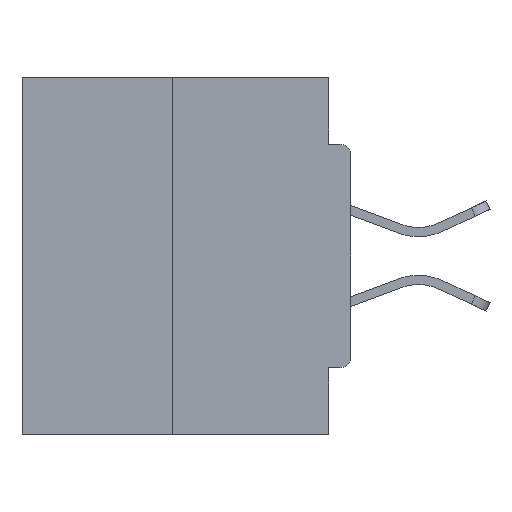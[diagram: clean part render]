
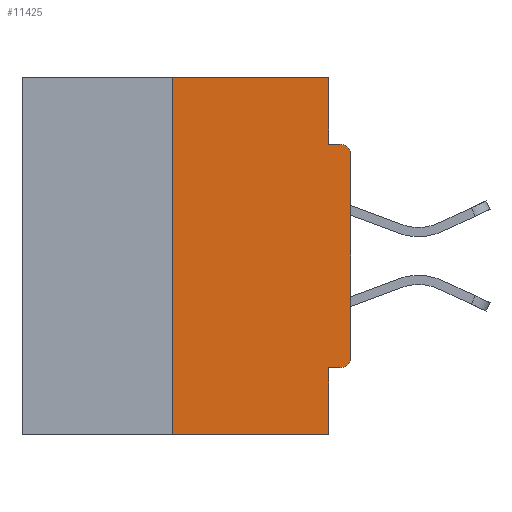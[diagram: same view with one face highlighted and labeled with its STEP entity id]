
A CAD part, left-side view. The second image highlights one B-rep face of the part: STEP entity #11425.
In plain terms, the highlighted planar face has unit normal (-1, 0, 0).
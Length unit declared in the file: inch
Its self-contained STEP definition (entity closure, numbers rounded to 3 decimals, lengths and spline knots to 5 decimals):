
#90 = VECTOR ( 'NONE', #6408, 39.37008 ) ;
#317 = ORIENTED_EDGE ( 'NONE', *, *, #34206, .F. ) ;
#780 = CARTESIAN_POINT ( 'NONE',  ( 0., 0.46, -0.5 ) ) ;
#1138 = VERTEX_POINT ( 'NONE', #7384 ) ;
#1147 = ORIENTED_EDGE ( 'NONE', *, *, #26222, .F. ) ;
#1891 = DIRECTION ( 'NONE',  ( 0., 0., 1. ) ) ;
#2937 = ORIENTED_EDGE ( 'NONE', *, *, #33532, .F. ) ;
#2979 = CARTESIAN_POINT ( 'NONE',  ( 0., 0.031, 0. ) ) ;
#3731 = LINE ( 'NONE', #7163, #4627 ) ;
#4180 = CARTESIAN_POINT ( 'NONE',  ( 0., 0.25, 0. ) ) ;
#4627 = VECTOR ( 'NONE', #1891, 39.37008 ) ;
#4870 = CARTESIAN_POINT ( 'NONE',  ( 0., 0.031, -0.4065 ) ) ;
#6396 = CARTESIAN_POINT ( 'NONE',  ( 0., 0.25, 0. ) ) ;
#6408 = DIRECTION ( 'NONE',  ( 0., -1., 0. ) ) ;
#6443 = DIRECTION ( 'NONE',  ( -1., 0., 0. ) ) ;
#6802 = DIRECTION ( 'NONE',  ( -1., 0., 0. ) ) ;
#7076 = VECTOR ( 'NONE', #23935, 39.37008 ) ;
#7163 = CARTESIAN_POINT ( 'NONE',  ( 0., 0., 0. ) ) ;
#7384 = CARTESIAN_POINT ( 'NONE',  ( 0., 0.25, -0.5 ) ) ;
#7463 = VECTOR ( 'NONE', #34844, 39.37008 ) ;
#7522 = LINE ( 'NONE', #31357, #90 ) ;
#7683 = ORIENTED_EDGE ( 'NONE', *, *, #14122, .T. ) ;
#8626 = EDGE_LOOP ( 'NONE', ( #9419, #317, #7683, #2937, #1147, #29762, #15945, #11208, #21785, #34174 ) ) ;
#8870 = EDGE_CURVE ( 'NONE', #30304, #31347, #3731, .T. ) ;
#8984 = CARTESIAN_POINT ( 'NONE',  ( 0., 0.031, -0.5 ) ) ;
#9339 = DIRECTION ( 'NONE',  ( 0., -1., 0. ) ) ;
#9419 = ORIENTED_EDGE ( 'NONE', *, *, #9723, .F. ) ;
#9717 = PLANE ( 'NONE',  #11985 ) ;
#9723 = EDGE_CURVE ( 'NONE', #26478, #11800, #12418, .T. ) ;
#10567 = CARTESIAN_POINT ( 'NONE',  ( 0., 0., -0.1085 ) ) ;
#10969 = CARTESIAN_POINT ( 'NONE',  ( 0., 0.015, -0.4065 ) ) ;
#10970 = LINE ( 'NONE', #30749, #25706 ) ;
#11057 = VERTEX_POINT ( 'NONE', #23684 ) ;
#11165 = VERTEX_POINT ( 'NONE', #10969 ) ;
#11208 = ORIENTED_EDGE ( 'NONE', *, *, #15128, .T. ) ;
#11425 = ADVANCED_FACE ( 'NONE', ( #17236 ), #9717, .F. ) ;
#11610 = CARTESIAN_POINT ( 'NONE',  ( 0., 0.031, 0. ) ) ;
#11800 = VERTEX_POINT ( 'NONE', #2979 ) ;
#11930 = CARTESIAN_POINT ( 'NONE',  ( 0., 0.015, -0.1085 ) ) ;
#11985 = AXIS2_PLACEMENT_3D ( 'NONE', #29256, #34636, #34876 ) ;
#12418 = LINE ( 'NONE', #28863, #19386 ) ;
#13959 = VECTOR ( 'NONE', #22725, 39.37008 ) ;
#14076 = EDGE_CURVE ( 'NONE', #33112, #11057, #7522, .T. ) ;
#14096 = VERTEX_POINT ( 'NONE', #8984 ) ;
#14122 = EDGE_CURVE ( 'NONE', #1138, #14096, #26658, .T. ) ;
#15128 = EDGE_CURVE ( 'NONE', #31347, #11057, #35312, .T. ) ;
#15945 = ORIENTED_EDGE ( 'NONE', *, *, #8870, .T. ) ;
#17236 = FACE_OUTER_BOUND ( 'NONE', #8626, .T. ) ;
#17503 = DIRECTION ( 'NONE',  ( 0., 0., -1. ) ) ;
#19281 = VECTOR ( 'NONE', #9339, 39.37008 ) ;
#19386 = VECTOR ( 'NONE', #31204, 39.37008 ) ;
#20306 = AXIS2_PLACEMENT_3D ( 'NONE', #11930, #6443, #31748 ) ;
#21430 = LINE ( 'NONE', #29426, #7076 ) ;
#21785 = ORIENTED_EDGE ( 'NONE', *, *, #14076, .F. ) ;
#21982 = VERTEX_POINT ( 'NONE', #4870 ) ;
#22725 = DIRECTION ( 'NONE',  ( 0., 0., -1. ) ) ;
#23684 = CARTESIAN_POINT ( 'NONE',  ( 0., 0.015, -0.0935 ) ) ;
#23935 = DIRECTION ( 'NONE',  ( 0., 0., -1. ) ) ;
#25668 = LINE ( 'NONE', #11610, #13959 ) ;
#25706 = VECTOR ( 'NONE', #30257, 39.37008 ) ;
#26222 = EDGE_CURVE ( 'NONE', #11165, #21982, #10970, .T. ) ;
#26478 = VERTEX_POINT ( 'NONE', #6396 ) ;
#26658 = LINE ( 'NONE', #780, #19281 ) ;
#27040 = EDGE_CURVE ( 'NONE', #11800, #33112, #25668, .T. ) ;
#27486 = LINE ( 'NONE', #4180, #7463 ) ;
#28863 = CARTESIAN_POINT ( 'NONE',  ( 0., 0.46, 0. ) ) ;
#29256 = CARTESIAN_POINT ( 'NONE',  ( 0., 0.46, 0. ) ) ;
#29426 = CARTESIAN_POINT ( 'NONE',  ( 0., 0.031, -0.5 ) ) ;
#29762 = ORIENTED_EDGE ( 'NONE', *, *, #33469, .T. ) ;
#30257 = DIRECTION ( 'NONE',  ( 0., 1., 0. ) ) ;
#30304 = VERTEX_POINT ( 'NONE', #34172 ) ;
#30454 = CARTESIAN_POINT ( 'NONE',  ( 0., 0.031, -0.0935 ) ) ;
#30676 = AXIS2_PLACEMENT_3D ( 'NONE', #31400, #6802, #17503 ) ;
#30749 = CARTESIAN_POINT ( 'NONE',  ( 0., 0., -0.4065 ) ) ;
#31204 = DIRECTION ( 'NONE',  ( 0., -1., 0. ) ) ;
#31347 = VERTEX_POINT ( 'NONE', #10567 ) ;
#31357 = CARTESIAN_POINT ( 'NONE',  ( 0., 0., -0.0935 ) ) ;
#31400 = CARTESIAN_POINT ( 'NONE',  ( 0., 0.015, -0.3915 ) ) ;
#31748 = DIRECTION ( 'NONE',  ( 0., 0., -1. ) ) ;
#33112 = VERTEX_POINT ( 'NONE', #30454 ) ;
#33469 = EDGE_CURVE ( 'NONE', #11165, #30304, #34505, .T. ) ;
#33532 = EDGE_CURVE ( 'NONE', #21982, #14096, #21430, .T. ) ;
#34172 = CARTESIAN_POINT ( 'NONE',  ( 0., 0., -0.3915 ) ) ;
#34174 = ORIENTED_EDGE ( 'NONE', *, *, #27040, .F. ) ;
#34206 = EDGE_CURVE ( 'NONE', #1138, #26478, #27486, .T. ) ;
#34505 = CIRCLE ( 'NONE', #30676, 0.015 ) ;
#34636 = DIRECTION ( 'NONE',  ( 1., 0., 0. ) ) ;
#34844 = DIRECTION ( 'NONE',  ( 0., 0., 1. ) ) ;
#34876 = DIRECTION ( 'NONE',  ( 0., 0., -1. ) ) ;
#35312 = CIRCLE ( 'NONE', #20306, 0.015 ) ;
